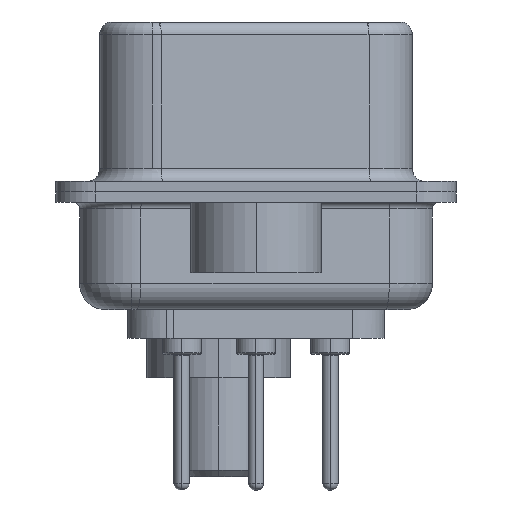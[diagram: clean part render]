
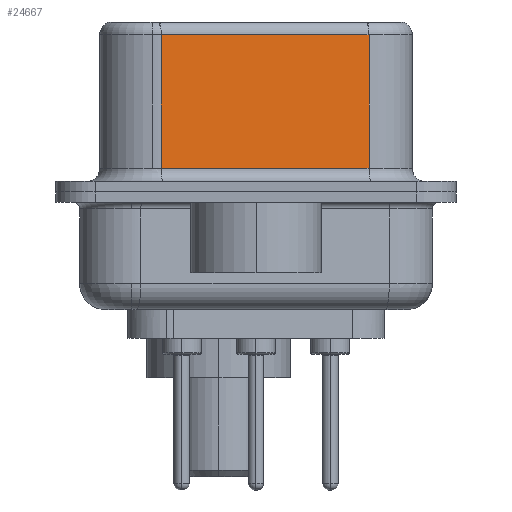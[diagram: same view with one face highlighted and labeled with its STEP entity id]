
A CAD part, left-side view. The second image highlights one B-rep face of the part: STEP entity #24667.
In plain terms, the highlighted planar face has unit normal (-0.985, -0.174, 0).
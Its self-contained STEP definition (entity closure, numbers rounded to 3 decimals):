
#647 = DIRECTION ( 'NONE',  ( 0.174, -0.985, 0. ) ) ;
#1687 = VECTOR ( 'NONE', #25658, 1000. ) ;
#3476 = CARTESIAN_POINT ( 'NONE',  ( 5.132, -4.322, 0.9 ) ) ;
#3546 = AXIS2_PLACEMENT_3D ( 'NONE', #16712, #3566, #18912 ) ;
#3566 = DIRECTION ( 'NONE',  ( 0.985, 0.174, 0. ) ) ;
#4322 = LINE ( 'NONE', #20145, #27084 ) ;
#4805 = ORIENTED_EDGE ( 'NONE', *, *, #14998, .T. ) ;
#5174 = ORIENTED_EDGE ( 'NONE', *, *, #11341, .F. ) ;
#6669 = LINE ( 'NONE', #19398, #23561 ) ;
#7910 = VERTEX_POINT ( 'NONE', #3476 ) ;
#8742 = VERTEX_POINT ( 'NONE', #26938 ) ;
#10262 = CARTESIAN_POINT ( 'NONE',  ( 5.132, -4.322, 6.02 ) ) ;
#11334 = CARTESIAN_POINT ( 'NONE',  ( 5.132, -4.322, 6.52 ) ) ;
#11341 = EDGE_CURVE ( 'NONE', #22965, #7910, #19903, .T. ) ;
#11389 = DIRECTION ( 'NONE',  ( -0.174, 0.985, 0. ) ) ;
#11601 = CARTESIAN_POINT ( 'NONE',  ( 5.132, -4.322, 0.9 ) ) ;
#12560 = CARTESIAN_POINT ( 'NONE',  ( 3.73, 3.628, 0.9 ) ) ;
#13205 = VECTOR ( 'NONE', #647, 1000. ) ;
#14998 = EDGE_CURVE ( 'NONE', #27886, #7910, #19748, .T. ) ;
#16712 = CARTESIAN_POINT ( 'NONE',  ( 5.132, -4.322, 6.52 ) ) ;
#18315 = EDGE_LOOP ( 'NONE', ( #5174, #20523, #22781, #4805 ) ) ;
#18912 = DIRECTION ( 'NONE',  ( -0.174, 0.985, 0. ) ) ;
#19398 = CARTESIAN_POINT ( 'NONE',  ( 3.73, 3.628, 6.52 ) ) ;
#19748 = LINE ( 'NONE', #11601, #13205 ) ;
#19903 = LINE ( 'NONE', #11334, #1687 ) ;
#20145 = CARTESIAN_POINT ( 'NONE',  ( 5.132, -4.322, 6.02 ) ) ;
#20382 = EDGE_CURVE ( 'NONE', #22965, #8742, #4322, .T. ) ;
#20523 = ORIENTED_EDGE ( 'NONE', *, *, #20382, .T. ) ;
#21732 = DIRECTION ( 'NONE',  ( 0., 0., -1. ) ) ;
#22190 = FACE_OUTER_BOUND ( 'NONE', #18315, .T. ) ;
#22498 = EDGE_CURVE ( 'NONE', #8742, #27886, #6669, .T. ) ;
#22781 = ORIENTED_EDGE ( 'NONE', *, *, #22498, .T. ) ;
#22965 = VERTEX_POINT ( 'NONE', #10262 ) ;
#23211 = PLANE ( 'NONE',  #3546 ) ;
#23561 = VECTOR ( 'NONE', #21732, 1000. ) ;
#24667 = ADVANCED_FACE ( 'NONE', ( #22190 ), #23211, .F. ) ;
#25658 = DIRECTION ( 'NONE',  ( 0., 0., -1. ) ) ;
#26938 = CARTESIAN_POINT ( 'NONE',  ( 3.73, 3.628, 6.02 ) ) ;
#27084 = VECTOR ( 'NONE', #11389, 1000. ) ;
#27886 = VERTEX_POINT ( 'NONE', #12560 ) ;
